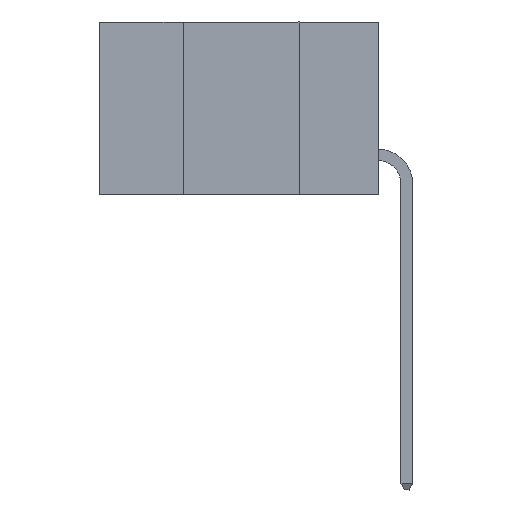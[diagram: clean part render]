
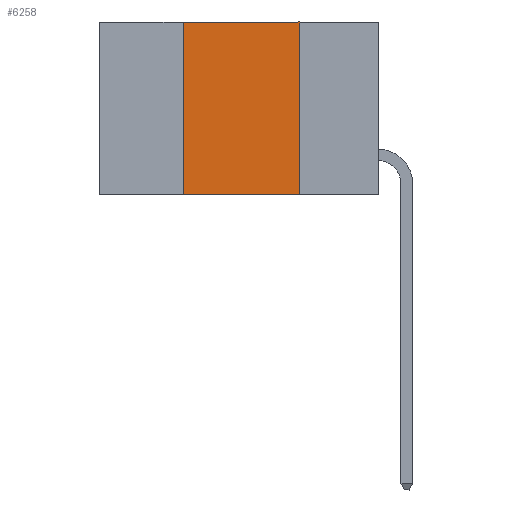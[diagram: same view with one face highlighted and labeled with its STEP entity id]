
A CAD part, left-side view. The second image highlights one B-rep face of the part: STEP entity #6258.
In plain terms, the highlighted planar face has unit normal (-1, 0, 0).
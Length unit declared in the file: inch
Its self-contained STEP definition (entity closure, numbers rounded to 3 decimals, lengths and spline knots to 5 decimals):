
#219 = DIRECTION ( 'NONE',  ( 0., 0., -1. ) ) ;
#911 = LINE ( 'NONE', #10425, #5336 ) ;
#940 = EDGE_CURVE ( 'NONE', #7830, #10629, #8172, .T. ) ;
#1037 = ORIENTED_EDGE ( 'NONE', *, *, #6304, .F. ) ;
#1248 = EDGE_LOOP ( 'NONE', ( #2867, #1037, #5260, #2262 ) ) ;
#1489 = AXIS2_PLACEMENT_3D ( 'NONE', #9025, #3641, #11020 ) ;
#1838 = VERTEX_POINT ( 'NONE', #10598 ) ;
#2262 = ORIENTED_EDGE ( 'NONE', *, *, #940, .T. ) ;
#2365 = EDGE_CURVE ( 'NONE', #1838, #10629, #911, .T. ) ;
#2415 = DIRECTION ( 'NONE',  ( 0., -1., 0. ) ) ;
#2867 = ORIENTED_EDGE ( 'NONE', *, *, #2365, .F. ) ;
#3109 = VECTOR ( 'NONE', #4522, 39.37008 ) ;
#3172 = LINE ( 'NONE', #7949, #4081 ) ;
#3524 = CARTESIAN_POINT ( 'NONE',  ( 0., 0.6, -0.37 ) ) ;
#3641 = DIRECTION ( 'NONE',  ( 1., 0., 0. ) ) ;
#4081 = VECTOR ( 'NONE', #5273, 39.37008 ) ;
#4522 = DIRECTION ( 'NONE',  ( 0., -1., 0. ) ) ;
#4525 = LINE ( 'NONE', #6339, #6398 ) ;
#5260 = ORIENTED_EDGE ( 'NONE', *, *, #9242, .F. ) ;
#5273 = DIRECTION ( 'NONE',  ( 0., 0., 1. ) ) ;
#5336 = VECTOR ( 'NONE', #219, 39.37008 ) ;
#5485 = VERTEX_POINT ( 'NONE', #7281 ) ;
#6258 = ADVANCED_FACE ( 'NONE', ( #10083 ), #10137, .F. ) ;
#6304 = EDGE_CURVE ( 'NONE', #5485, #1838, #4525, .T. ) ;
#6339 = CARTESIAN_POINT ( 'NONE',  ( 0., 0.6, 0. ) ) ;
#6398 = VECTOR ( 'NONE', #2415, 39.37008 ) ;
#6771 = CARTESIAN_POINT ( 'NONE',  ( 0., 0.42, -0.37 ) ) ;
#7281 = CARTESIAN_POINT ( 'NONE',  ( 0., 0.42, 0. ) ) ;
#7830 = VERTEX_POINT ( 'NONE', #6771 ) ;
#7949 = CARTESIAN_POINT ( 'NONE',  ( 0., 0.42, -0.37 ) ) ;
#8172 = LINE ( 'NONE', #3524, #3109 ) ;
#9025 = CARTESIAN_POINT ( 'NONE',  ( 0., 0.6, 0. ) ) ;
#9242 = EDGE_CURVE ( 'NONE', #7830, #5485, #3172, .T. ) ;
#9815 = CARTESIAN_POINT ( 'NONE',  ( 0., 0.17, -0.37 ) ) ;
#10083 = FACE_OUTER_BOUND ( 'NONE', #1248, .T. ) ;
#10137 = PLANE ( 'NONE',  #1489 ) ;
#10425 = CARTESIAN_POINT ( 'NONE',  ( 0., 0.17, -0.37 ) ) ;
#10598 = CARTESIAN_POINT ( 'NONE',  ( 0., 0.17, 0. ) ) ;
#10629 = VERTEX_POINT ( 'NONE', #9815 ) ;
#11020 = DIRECTION ( 'NONE',  ( 0., 0., -1. ) ) ;
